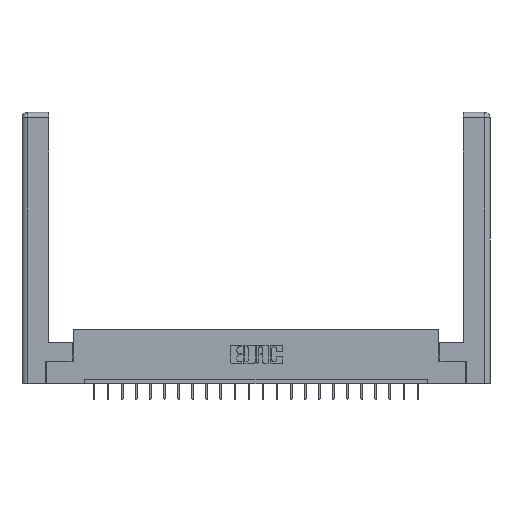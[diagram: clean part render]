
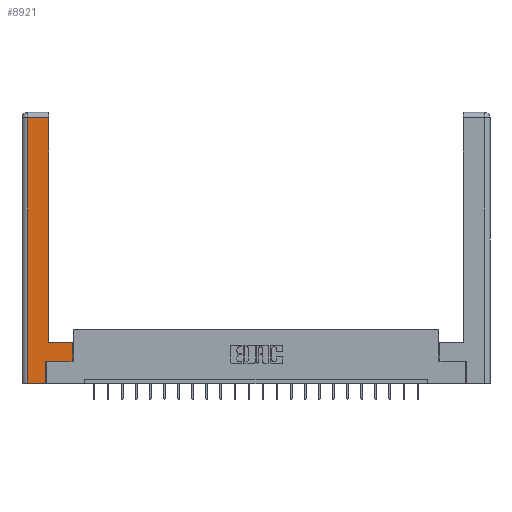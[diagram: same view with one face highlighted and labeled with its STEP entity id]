
A CAD part, top view. The second image highlights one B-rep face of the part: STEP entity #8921.
In plain terms, the highlighted planar face has unit normal (0, 0, 1).
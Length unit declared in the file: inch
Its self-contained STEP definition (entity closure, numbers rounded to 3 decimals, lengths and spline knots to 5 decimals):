
#217 = LINE ( 'NONE', #9097, #10158 ) ;
#558 = EDGE_CURVE ( 'NONE', #16194, #14105, #11984, .T. ) ;
#1065 = CARTESIAN_POINT ( 'NONE',  ( 0.295, 0.45, 0. ) ) ;
#1247 = DIRECTION ( 'NONE',  ( 0., 1., 0. ) ) ;
#1422 = CARTESIAN_POINT ( 'NONE',  ( 0.265, 0.245, 0. ) ) ;
#1988 = ORIENTED_EDGE ( 'NONE', *, *, #13877, .T. ) ;
#2249 = EDGE_CURVE ( 'NONE', #12203, #18703, #8015, .T. ) ;
#2326 = ORIENTED_EDGE ( 'NONE', *, *, #6800, .T. ) ;
#3324 = LINE ( 'NONE', #15818, #5801 ) ;
#3361 = DIRECTION ( 'NONE',  ( 0., 1., 0. ) ) ;
#3613 = CARTESIAN_POINT ( 'NONE',  ( 0.265, 0., 0. ) ) ;
#4277 = EDGE_CURVE ( 'NONE', #14105, #4816, #7142, .T. ) ;
#4816 = VERTEX_POINT ( 'NONE', #4934 ) ;
#4850 = FACE_OUTER_BOUND ( 'NONE', #15359, .T. ) ;
#4934 = CARTESIAN_POINT ( 'NONE',  ( 0.295, 2.94, 0. ) ) ;
#5396 = EDGE_CURVE ( 'NONE', #9956, #12203, #7304, .T. ) ;
#5464 = ORIENTED_EDGE ( 'NONE', *, *, #15253, .T. ) ;
#5801 = VECTOR ( 'NONE', #7072, 39.37008 ) ;
#5983 = PLANE ( 'NONE',  #15896 ) ;
#6800 = EDGE_CURVE ( 'NONE', #13645, #16194, #15160, .T. ) ;
#7072 = DIRECTION ( 'NONE',  ( 1., 0., 0. ) ) ;
#7142 = LINE ( 'NONE', #8645, #9039 ) ;
#7304 = LINE ( 'NONE', #17191, #21341 ) ;
#7772 = CARTESIAN_POINT ( 'NONE',  ( 0.295, 0.45, 0. ) ) ;
#7811 = CARTESIAN_POINT ( 'NONE',  ( 0.265, 0., 0. ) ) ;
#8015 = LINE ( 'NONE', #7811, #14115 ) ;
#8496 = DIRECTION ( 'NONE',  ( 0., -1., 0. ) ) ;
#8645 = CARTESIAN_POINT ( 'NONE',  ( 0.295, 3., 0. ) ) ;
#8759 = VECTOR ( 'NONE', #1247, 39.37008 ) ;
#8786 = DIRECTION ( 'NONE',  ( -1., 0., 0. ) ) ;
#8921 = ADVANCED_FACE ( 'NONE', ( #4850 ), #5983, .F. ) ;
#9039 = VECTOR ( 'NONE', #3361, 39.37008 ) ;
#9097 = CARTESIAN_POINT ( 'NONE',  ( 0.0615, 2.94, 0. ) ) ;
#9373 = CARTESIAN_POINT ( 'NONE',  ( 0., 0., 0. ) ) ;
#9592 = ORIENTED_EDGE ( 'NONE', *, *, #2249, .T. ) ;
#9956 = VERTEX_POINT ( 'NONE', #22553 ) ;
#9958 = ORIENTED_EDGE ( 'NONE', *, *, #5396, .T. ) ;
#10158 = VECTOR ( 'NONE', #8786, 39.37008 ) ;
#10304 = VECTOR ( 'NONE', #15046, 39.37008 ) ;
#11165 = CARTESIAN_POINT ( 'NONE',  ( 0.0615, 0., 0. ) ) ;
#11363 = CARTESIAN_POINT ( 'NONE',  ( 0.265, 0.245, 0. ) ) ;
#11984 = LINE ( 'NONE', #1065, #10304 ) ;
#12203 = VERTEX_POINT ( 'NONE', #11165 ) ;
#12494 = LINE ( 'NONE', #1422, #14446 ) ;
#12499 = EDGE_CURVE ( 'NONE', #18703, #22604, #12494, .T. ) ;
#12953 = DIRECTION ( 'NONE',  ( -1., 0., 0. ) ) ;
#13081 = DIRECTION ( 'NONE',  ( 1., 0., 0. ) ) ;
#13415 = CARTESIAN_POINT ( 'NONE',  ( 0.565, 0.45, 0. ) ) ;
#13560 = DIRECTION ( 'NONE',  ( 0., 1., 0. ) ) ;
#13645 = VERTEX_POINT ( 'NONE', #20990 ) ;
#13877 = EDGE_CURVE ( 'NONE', #22604, #13645, #3324, .T. ) ;
#14105 = VERTEX_POINT ( 'NONE', #7772 ) ;
#14115 = VECTOR ( 'NONE', #13081, 39.37008 ) ;
#14446 = VECTOR ( 'NONE', #13560, 39.37008 ) ;
#15046 = DIRECTION ( 'NONE',  ( -1., 0., 0. ) ) ;
#15160 = LINE ( 'NONE', #20639, #8759 ) ;
#15253 = EDGE_CURVE ( 'NONE', #4816, #9956, #217, .T. ) ;
#15359 = EDGE_LOOP ( 'NONE', ( #17509, #5464, #9958, #9592, #15628, #1988, #2326, #21806 ) ) ;
#15628 = ORIENTED_EDGE ( 'NONE', *, *, #12499, .T. ) ;
#15818 = CARTESIAN_POINT ( 'NONE',  ( 0.565, 0.245, 0. ) ) ;
#15896 = AXIS2_PLACEMENT_3D ( 'NONE', #9373, #21749, #12953 ) ;
#16194 = VERTEX_POINT ( 'NONE', #13415 ) ;
#17191 = CARTESIAN_POINT ( 'NONE',  ( 0.0615, 0., 0. ) ) ;
#17509 = ORIENTED_EDGE ( 'NONE', *, *, #4277, .T. ) ;
#18703 = VERTEX_POINT ( 'NONE', #3613 ) ;
#20639 = CARTESIAN_POINT ( 'NONE',  ( 0.565, 0.45, 0. ) ) ;
#20990 = CARTESIAN_POINT ( 'NONE',  ( 0.565, 0.245, 0. ) ) ;
#21341 = VECTOR ( 'NONE', #8496, 39.37008 ) ;
#21749 = DIRECTION ( 'NONE',  ( 0., 0., -1. ) ) ;
#21806 = ORIENTED_EDGE ( 'NONE', *, *, #558, .T. ) ;
#22553 = CARTESIAN_POINT ( 'NONE',  ( 0.0615, 2.94, 0. ) ) ;
#22604 = VERTEX_POINT ( 'NONE', #11363 ) ;
